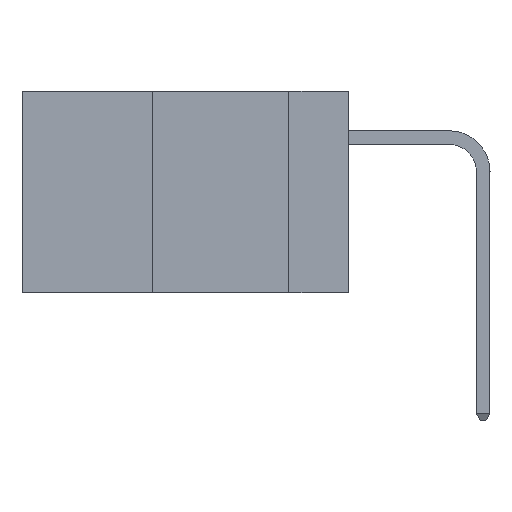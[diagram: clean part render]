
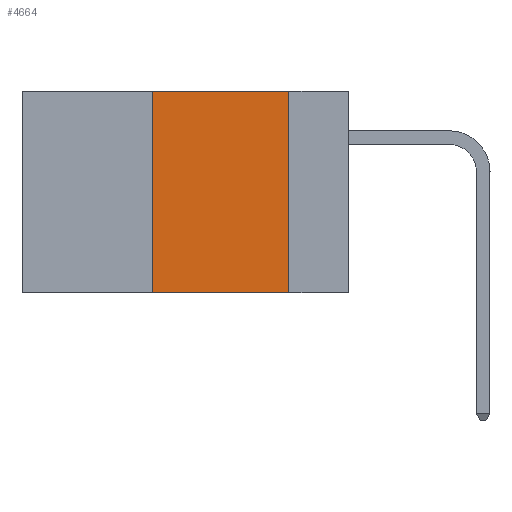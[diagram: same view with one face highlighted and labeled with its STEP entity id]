
A CAD part, left-side view. The second image highlights one B-rep face of the part: STEP entity #4664.
In plain terms, the highlighted planar face has unit normal (-1, 0, 0).
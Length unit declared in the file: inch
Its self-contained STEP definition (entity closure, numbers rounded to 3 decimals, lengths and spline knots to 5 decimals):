
#1129 = VECTOR ( 'NONE', #12229, 39.37008 ) ;
#1421 = VECTOR ( 'NONE', #11372, 39.37008 ) ;
#1870 = LINE ( 'NONE', #7744, #1129 ) ;
#1880 = ORIENTED_EDGE ( 'NONE', *, *, #10504, .F. ) ;
#2048 = CARTESIAN_POINT ( 'NONE',  ( 0., 0.11, 0. ) ) ;
#2561 = EDGE_CURVE ( 'NONE', #3698, #12821, #14041, .T. ) ;
#3056 = AXIS2_PLACEMENT_3D ( 'NONE', #12017, #7044, #10965 ) ;
#3658 = VERTEX_POINT ( 'NONE', #7414 ) ;
#3698 = VERTEX_POINT ( 'NONE', #7248 ) ;
#4038 = VECTOR ( 'NONE', #7748, 39.37008 ) ;
#4664 = ADVANCED_FACE ( 'NONE', ( #11484 ), #11972, .F. ) ;
#4756 = EDGE_CURVE ( 'NONE', #3698, #3658, #10423, .T. ) ;
#5224 = ORIENTED_EDGE ( 'NONE', *, *, #12221, .F. ) ;
#5272 = VECTOR ( 'NONE', #6515, 39.37008 ) ;
#5534 = CARTESIAN_POINT ( 'NONE',  ( 0., 0.11, 0. ) ) ;
#6395 = CARTESIAN_POINT ( 'NONE',  ( 0., 0.6, -0.37 ) ) ;
#6515 = DIRECTION ( 'NONE',  ( 0., -1., 0. ) ) ;
#6757 = ORIENTED_EDGE ( 'NONE', *, *, #4756, .F. ) ;
#6991 = LINE ( 'NONE', #5534, #4038 ) ;
#7044 = DIRECTION ( 'NONE',  ( 1., 0., 0. ) ) ;
#7248 = CARTESIAN_POINT ( 'NONE',  ( 0., 0.36, -0.37 ) ) ;
#7414 = CARTESIAN_POINT ( 'NONE',  ( 0., 0.36, 0. ) ) ;
#7744 = CARTESIAN_POINT ( 'NONE',  ( 0., 0.6, 0. ) ) ;
#7748 = DIRECTION ( 'NONE',  ( 0., 0., -1. ) ) ;
#7969 = ORIENTED_EDGE ( 'NONE', *, *, #2561, .T. ) ;
#8712 = VERTEX_POINT ( 'NONE', #2048 ) ;
#10423 = LINE ( 'NONE', #11422, #1421 ) ;
#10504 = EDGE_CURVE ( 'NONE', #3658, #8712, #1870, .T. ) ;
#10965 = DIRECTION ( 'NONE',  ( 0., 0., -1. ) ) ;
#11372 = DIRECTION ( 'NONE',  ( 0., 0., 1. ) ) ;
#11422 = CARTESIAN_POINT ( 'NONE',  ( 0., 0.36, 0. ) ) ;
#11484 = FACE_OUTER_BOUND ( 'NONE', #12075, .T. ) ;
#11972 = PLANE ( 'NONE',  #3056 ) ;
#12017 = CARTESIAN_POINT ( 'NONE',  ( 0., 0.6, 0. ) ) ;
#12075 = EDGE_LOOP ( 'NONE', ( #5224, #1880, #6757, #7969 ) ) ;
#12221 = EDGE_CURVE ( 'NONE', #8712, #12821, #6991, .T. ) ;
#12229 = DIRECTION ( 'NONE',  ( 0., -1., 0. ) ) ;
#12821 = VERTEX_POINT ( 'NONE', #13956 ) ;
#13956 = CARTESIAN_POINT ( 'NONE',  ( 0., 0.11, -0.37 ) ) ;
#14041 = LINE ( 'NONE', #6395, #5272 ) ;
